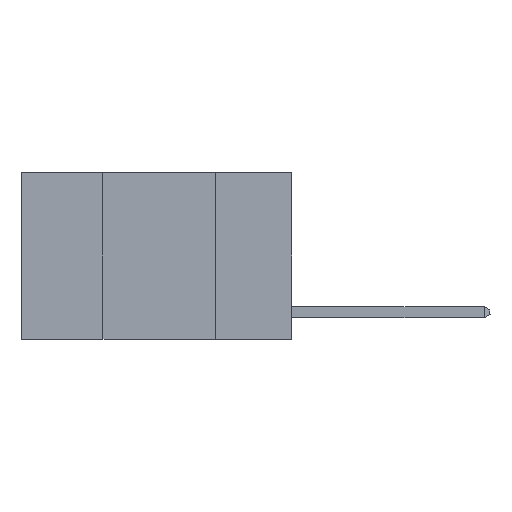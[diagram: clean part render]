
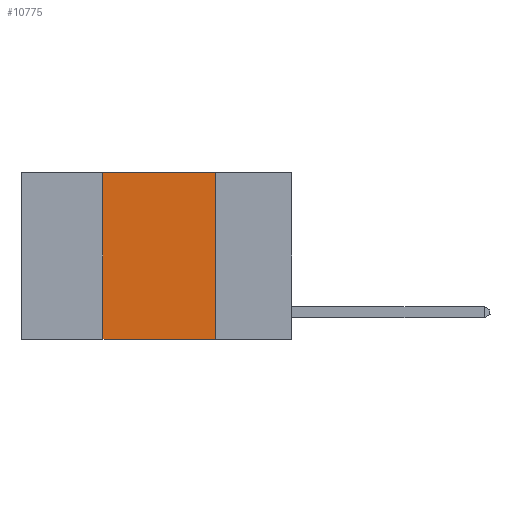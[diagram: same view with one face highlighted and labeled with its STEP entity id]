
A CAD part, left-side view. The second image highlights one B-rep face of the part: STEP entity #10775.
In plain terms, the highlighted planar face has unit normal (-1, 0, 0).
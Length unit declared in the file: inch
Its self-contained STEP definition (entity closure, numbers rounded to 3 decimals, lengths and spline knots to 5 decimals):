
#443 = EDGE_CURVE ( 'NONE', #4382, #9093, #10247, .T. ) ;
#562 = FACE_OUTER_BOUND ( 'NONE', #12859, .T. ) ;
#1156 = DIRECTION ( 'NONE',  ( 0., -1., 0. ) ) ;
#1344 = LINE ( 'NONE', #5670, #11612 ) ;
#2031 = EDGE_CURVE ( 'NONE', #8587, #13072, #7137, .T. ) ;
#2252 = DIRECTION ( 'NONE',  ( 0., 0., 1. ) ) ;
#3351 = CARTESIAN_POINT ( 'NONE',  ( 0., 0.17, 0. ) ) ;
#4382 = VERTEX_POINT ( 'NONE', #6570 ) ;
#5174 = PLANE ( 'NONE',  #6280 ) ;
#5670 = CARTESIAN_POINT ( 'NONE',  ( 0., 0.42, 0. ) ) ;
#6099 = EDGE_CURVE ( 'NONE', #13072, #9093, #13783, .T. ) ;
#6147 = DIRECTION ( 'NONE',  ( 1., 0., 0. ) ) ;
#6280 = AXIS2_PLACEMENT_3D ( 'NONE', #9520, #6147, #13184 ) ;
#6396 = ORIENTED_EDGE ( 'NONE', *, *, #2031, .F. ) ;
#6570 = CARTESIAN_POINT ( 'NONE',  ( 0., 0.42, -0.37 ) ) ;
#6882 = ORIENTED_EDGE ( 'NONE', *, *, #6099, .F. ) ;
#7062 = CARTESIAN_POINT ( 'NONE',  ( 0., 0.6, 0. ) ) ;
#7137 = LINE ( 'NONE', #7062, #8073 ) ;
#8073 = VECTOR ( 'NONE', #8330, 39.37008 ) ;
#8330 = DIRECTION ( 'NONE',  ( 0., -1., 0. ) ) ;
#8587 = VERTEX_POINT ( 'NONE', #12172 ) ;
#9093 = VERTEX_POINT ( 'NONE', #14420 ) ;
#9520 = CARTESIAN_POINT ( 'NONE',  ( 0., 0.6, 0. ) ) ;
#9918 = ORIENTED_EDGE ( 'NONE', *, *, #443, .T. ) ;
#10175 = CARTESIAN_POINT ( 'NONE',  ( 0., 0.6, -0.37 ) ) ;
#10247 = LINE ( 'NONE', #10175, #12057 ) ;
#10775 = ADVANCED_FACE ( 'NONE', ( #562 ), #5174, .F. ) ;
#11612 = VECTOR ( 'NONE', #2252, 39.37008 ) ;
#12057 = VECTOR ( 'NONE', #1156, 39.37008 ) ;
#12172 = CARTESIAN_POINT ( 'NONE',  ( 0., 0.42, 0. ) ) ;
#12706 = EDGE_CURVE ( 'NONE', #4382, #8587, #1344, .T. ) ;
#12859 = EDGE_LOOP ( 'NONE', ( #6882, #6396, #13095, #9918 ) ) ;
#12892 = CARTESIAN_POINT ( 'NONE',  ( 0., 0.17, 0. ) ) ;
#13072 = VERTEX_POINT ( 'NONE', #3351 ) ;
#13095 = ORIENTED_EDGE ( 'NONE', *, *, #12706, .F. ) ;
#13184 = DIRECTION ( 'NONE',  ( 0., 0., -1. ) ) ;
#13783 = LINE ( 'NONE', #12892, #14408 ) ;
#13861 = DIRECTION ( 'NONE',  ( 0., 0., -1. ) ) ;
#14408 = VECTOR ( 'NONE', #13861, 39.37008 ) ;
#14420 = CARTESIAN_POINT ( 'NONE',  ( 0., 0.17, -0.37 ) ) ;
